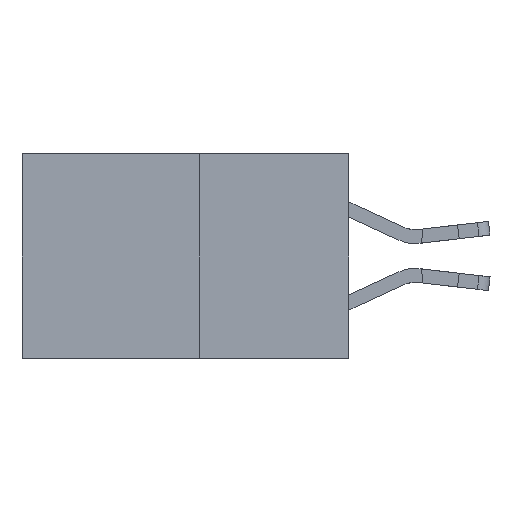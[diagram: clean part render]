
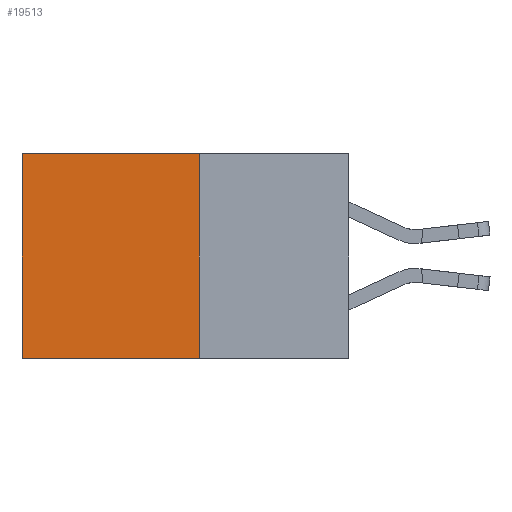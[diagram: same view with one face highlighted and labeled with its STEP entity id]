
A CAD part, left-side view. The second image highlights one B-rep face of the part: STEP entity #19513.
In plain terms, the highlighted planar face has unit normal (-1, 0, 0).
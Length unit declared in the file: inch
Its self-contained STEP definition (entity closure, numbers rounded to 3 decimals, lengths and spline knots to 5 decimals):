
#124 = VERTEX_POINT ( 'NONE', #3537 ) ;
#1463 = ORIENTED_EDGE ( 'NONE', *, *, #17692, .T. ) ;
#2549 = LINE ( 'NONE', #24832, #22657 ) ;
#3537 = CARTESIAN_POINT ( 'NONE',  ( 0.277, 0.59, 0. ) ) ;
#3981 = CARTESIAN_POINT ( 'NONE',  ( 0.277, 0.27, 0. ) ) ;
#4140 = LINE ( 'NONE', #17152, #24186 ) ;
#4987 = LINE ( 'NONE', #11089, #19925 ) ;
#5641 = EDGE_CURVE ( 'NONE', #10080, #16491, #2549, .T. ) ;
#5847 = ORIENTED_EDGE ( 'NONE', *, *, #5641, .F. ) ;
#6217 = CARTESIAN_POINT ( 'NONE',  ( 0.277, 0.59, -0.37 ) ) ;
#7429 = DIRECTION ( 'NONE',  ( 0., 0., -1. ) ) ;
#7965 = EDGE_LOOP ( 'NONE', ( #1463, #9421, #5847, #21460 ) ) ;
#8356 = DIRECTION ( 'NONE',  ( 0., 0., -1. ) ) ;
#9235 = DIRECTION ( 'NONE',  ( 0., 1., 0. ) ) ;
#9284 = AXIS2_PLACEMENT_3D ( 'NONE', #18081, #20020, #8356 ) ;
#9377 = DIRECTION ( 'NONE',  ( 0., 0., -1. ) ) ;
#9421 = ORIENTED_EDGE ( 'NONE', *, *, #12584, .F. ) ;
#10080 = VERTEX_POINT ( 'NONE', #3981 ) ;
#11089 = CARTESIAN_POINT ( 'NONE',  ( 0.277, 0.27, -0.37 ) ) ;
#12549 = CARTESIAN_POINT ( 'NONE',  ( 0.277, 0.27, 0. ) ) ;
#12584 = EDGE_CURVE ( 'NONE', #16491, #12979, #4987, .T. ) ;
#12979 = VERTEX_POINT ( 'NONE', #6217 ) ;
#15446 = VECTOR ( 'NONE', #22229, 39.37008 ) ;
#16106 = PLANE ( 'NONE',  #9284 ) ;
#16491 = VERTEX_POINT ( 'NONE', #25083 ) ;
#17152 = CARTESIAN_POINT ( 'NONE',  ( 0.277, 0.59, -0.37 ) ) ;
#17430 = EDGE_CURVE ( 'NONE', #10080, #124, #25089, .T. ) ;
#17692 = EDGE_CURVE ( 'NONE', #124, #12979, #4140, .T. ) ;
#18081 = CARTESIAN_POINT ( 'NONE',  ( 0.277, 0.27, -0.37 ) ) ;
#19016 = FACE_OUTER_BOUND ( 'NONE', #7965, .T. ) ;
#19513 = ADVANCED_FACE ( 'NONE', ( #19016 ), #16106, .F. ) ;
#19925 = VECTOR ( 'NONE', #9235, 39.37008 ) ;
#20020 = DIRECTION ( 'NONE',  ( 1., 0., 0. ) ) ;
#21460 = ORIENTED_EDGE ( 'NONE', *, *, #17430, .T. ) ;
#22229 = DIRECTION ( 'NONE',  ( 0., 1., 0. ) ) ;
#22657 = VECTOR ( 'NONE', #9377, 39.37008 ) ;
#24186 = VECTOR ( 'NONE', #7429, 39.37008 ) ;
#24832 = CARTESIAN_POINT ( 'NONE',  ( 0.277, 0.27, -0.37 ) ) ;
#25083 = CARTESIAN_POINT ( 'NONE',  ( 0.277, 0.27, -0.37 ) ) ;
#25089 = LINE ( 'NONE', #12549, #15446 ) ;
